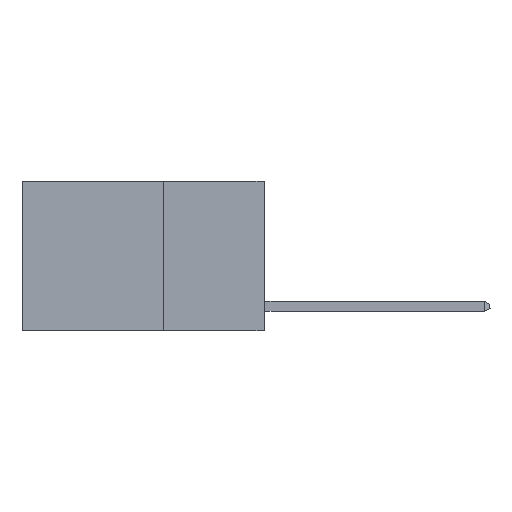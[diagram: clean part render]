
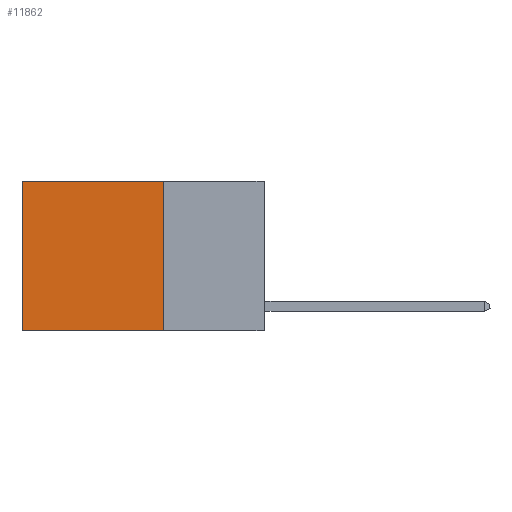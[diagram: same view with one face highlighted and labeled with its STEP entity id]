
A CAD part, left-side view. The second image highlights one B-rep face of the part: STEP entity #11862.
In plain terms, the highlighted planar face has unit normal (-1, 0, 0).
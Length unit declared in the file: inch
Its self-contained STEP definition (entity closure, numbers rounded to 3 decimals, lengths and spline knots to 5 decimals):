
#292 = LINE ( 'NONE', #2338, #4274 ) ;
#1362 = EDGE_CURVE ( 'NONE', #12942, #8414, #6692, .T. ) ;
#2215 = EDGE_CURVE ( 'NONE', #7651, #8414, #9383, .T. ) ;
#2338 = CARTESIAN_POINT ( 'NONE',  ( 0.2625, 0.25, 0. ) ) ;
#2351 = EDGE_LOOP ( 'NONE', ( #5945, #6954, #2965, #9997 ) ) ;
#2965 = ORIENTED_EDGE ( 'NONE', *, *, #12787, .F. ) ;
#3680 = VERTEX_POINT ( 'NONE', #12484 ) ;
#4274 = VECTOR ( 'NONE', #11180, 39.37008 ) ;
#4983 = DIRECTION ( 'NONE',  ( 0., 1., 0. ) ) ;
#5146 = VECTOR ( 'NONE', #18471, 39.37008 ) ;
#5504 = CARTESIAN_POINT ( 'NONE',  ( 0.2625, 0.25, -0.37 ) ) ;
#5766 = PLANE ( 'NONE',  #6685 ) ;
#5945 = ORIENTED_EDGE ( 'NONE', *, *, #2215, .T. ) ;
#6685 = AXIS2_PLACEMENT_3D ( 'NONE', #12970, #15832, #7268 ) ;
#6692 = LINE ( 'NONE', #5504, #13888 ) ;
#6954 = ORIENTED_EDGE ( 'NONE', *, *, #1362, .F. ) ;
#7143 = CARTESIAN_POINT ( 'NONE',  ( 0.2625, 0.25, -0.37 ) ) ;
#7268 = DIRECTION ( 'NONE',  ( 0., 0., -1. ) ) ;
#7443 = EDGE_CURVE ( 'NONE', #3680, #7651, #13312, .T. ) ;
#7651 = VERTEX_POINT ( 'NONE', #13252 ) ;
#8414 = VERTEX_POINT ( 'NONE', #13529 ) ;
#8426 = CARTESIAN_POINT ( 'NONE',  ( 0.2625, 0.6, 0. ) ) ;
#9358 = FACE_OUTER_BOUND ( 'NONE', #2351, .T. ) ;
#9383 = LINE ( 'NONE', #8426, #16519 ) ;
#9856 = DIRECTION ( 'NONE',  ( 0., 0., -1. ) ) ;
#9997 = ORIENTED_EDGE ( 'NONE', *, *, #7443, .T. ) ;
#11180 = DIRECTION ( 'NONE',  ( 0., 0., -1. ) ) ;
#11323 = CARTESIAN_POINT ( 'NONE',  ( 0.2625, 0.25, 0. ) ) ;
#11862 = ADVANCED_FACE ( 'NONE', ( #9358 ), #5766, .F. ) ;
#12484 = CARTESIAN_POINT ( 'NONE',  ( 0.2625, 0.25, 0. ) ) ;
#12787 = EDGE_CURVE ( 'NONE', #3680, #12942, #292, .T. ) ;
#12942 = VERTEX_POINT ( 'NONE', #7143 ) ;
#12970 = CARTESIAN_POINT ( 'NONE',  ( 0.2625, 0.25, 0. ) ) ;
#13252 = CARTESIAN_POINT ( 'NONE',  ( 0.2625, 0.6, 0. ) ) ;
#13312 = LINE ( 'NONE', #11323, #5146 ) ;
#13529 = CARTESIAN_POINT ( 'NONE',  ( 0.2625, 0.6, -0.37 ) ) ;
#13888 = VECTOR ( 'NONE', #4983, 39.37008 ) ;
#15832 = DIRECTION ( 'NONE',  ( 1., 0., 0. ) ) ;
#16519 = VECTOR ( 'NONE', #9856, 39.37008 ) ;
#18471 = DIRECTION ( 'NONE',  ( 0., 1., 0. ) ) ;
